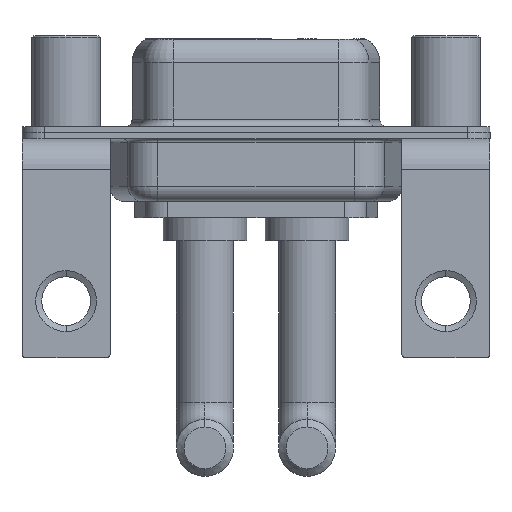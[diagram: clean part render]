
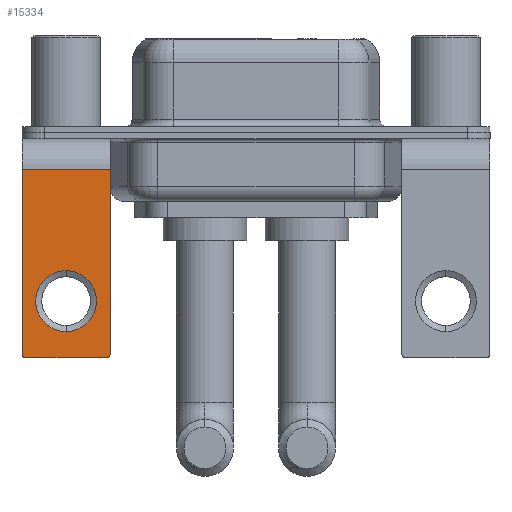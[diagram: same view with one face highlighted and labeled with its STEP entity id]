
A CAD part, front view. The second image highlights one B-rep face of the part: STEP entity #15334.
In plain terms, the highlighted planar face has unit normal (0, -1, 0).
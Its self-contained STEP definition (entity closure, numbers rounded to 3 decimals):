
#143 = CARTESIAN_POINT ( 'NONE',  ( -2.9, -6.25, -14.55 ) ) ;
#316 = CARTESIAN_POINT ( 'NONE',  ( 2.9, -6.25, -2.4 ) ) ;
#358 = ORIENTED_EDGE ( 'NONE', *, *, #3261, .T. ) ;
#514 = DIRECTION ( 'NONE',  ( 0., 0., 1. ) ) ;
#973 = VERTEX_POINT ( 'NONE', #11281 ) ;
#980 = CIRCLE ( 'NONE', #6092, 0.25 ) ;
#1314 = VECTOR ( 'NONE', #4201, 1000. ) ;
#1320 = VECTOR ( 'NONE', #4172, 1000. ) ;
#1619 = DIRECTION ( 'NONE',  ( -1., 0., 0. ) ) ;
#1634 = AXIS2_PLACEMENT_3D ( 'NONE', #6659, #12765, #7776 ) ;
#1833 = CARTESIAN_POINT ( 'NONE',  ( 0., -6.25, -11.07 ) ) ;
#1872 = CARTESIAN_POINT ( 'NONE',  ( -2.9, -6.25, -2.4 ) ) ;
#1983 = CARTESIAN_POINT ( 'NONE',  ( 2.65, -6.25, -14.8 ) ) ;
#2812 = VERTEX_POINT ( 'NONE', #143 ) ;
#3261 = EDGE_CURVE ( 'NONE', #2812, #8365, #980, .T. ) ;
#4140 = VECTOR ( 'NONE', #1619, 1000. ) ;
#4163 = FACE_BOUND ( 'NONE', #8714, .T. ) ;
#4172 = DIRECTION ( 'NONE',  ( 0., 0., -1. ) ) ;
#4201 = DIRECTION ( 'NONE',  ( -1., 0., 0. ) ) ;
#4545 = EDGE_CURVE ( 'NONE', #973, #2812, #15182, .T. ) ;
#4683 = AXIS2_PLACEMENT_3D ( 'NONE', #1833, #15303, #13061 ) ;
#4737 = EDGE_LOOP ( 'NONE', ( #15583, #358, #13802, #5341, #8383, #10522 ) ) ;
#4796 = DIRECTION ( 'NONE',  ( 0., -1., 0. ) ) ;
#5288 = EDGE_CURVE ( 'NONE', #7611, #15326, #15635, .T. ) ;
#5341 = ORIENTED_EDGE ( 'NONE', *, *, #14428, .T. ) ;
#5610 = EDGE_CURVE ( 'NONE', #14534, #8365, #6503, .T. ) ;
#5647 = EDGE_CURVE ( 'NONE', #5901, #12718, #8306, .T. ) ;
#5901 = VERTEX_POINT ( 'NONE', #11033 ) ;
#5910 = CARTESIAN_POINT ( 'NONE',  ( 2.9, -6.25, -14.55 ) ) ;
#5926 = CARTESIAN_POINT ( 'NONE',  ( 0., -6.25, -11.07 ) ) ;
#6048 = DIRECTION ( 'NONE',  ( 0., 0., -1. ) ) ;
#6092 = AXIS2_PLACEMENT_3D ( 'NONE', #9459, #4796, #14524 ) ;
#6503 = LINE ( 'NONE', #13732, #4140 ) ;
#6659 = CARTESIAN_POINT ( 'NONE',  ( 2.65, -6.25, -14.55 ) ) ;
#6834 = DIRECTION ( 'NONE',  ( 0., 1., 0. ) ) ;
#7110 = CARTESIAN_POINT ( 'NONE',  ( 0., -6.25, -9.07 ) ) ;
#7523 = ORIENTED_EDGE ( 'NONE', *, *, #5288, .T. ) ;
#7611 = VERTEX_POINT ( 'NONE', #7110 ) ;
#7776 = DIRECTION ( 'NONE',  ( 0., 0., 1. ) ) ;
#8037 = CIRCLE ( 'NONE', #4683, 2. ) ;
#8306 = LINE ( 'NONE', #9587, #15433 ) ;
#8365 = VERTEX_POINT ( 'NONE', #8973 ) ;
#8383 = ORIENTED_EDGE ( 'NONE', *, *, #5647, .F. ) ;
#8704 = AXIS2_PLACEMENT_3D ( 'NONE', #5926, #6834, #15500 ) ;
#8714 = EDGE_LOOP ( 'NONE', ( #12836, #7523 ) ) ;
#8802 = AXIS2_PLACEMENT_3D ( 'NONE', #9298, #11482, #514 ) ;
#8973 = CARTESIAN_POINT ( 'NONE',  ( -2.65, -6.25, -14.8 ) ) ;
#9298 = CARTESIAN_POINT ( 'NONE',  ( 2.9, -6.25, -2.4 ) ) ;
#9459 = CARTESIAN_POINT ( 'NONE',  ( -2.65, -6.25, -14.55 ) ) ;
#9587 = CARTESIAN_POINT ( 'NONE',  ( 2.9, -6.25, -2.4 ) ) ;
#9976 = EDGE_CURVE ( 'NONE', #5901, #973, #11442, .T. ) ;
#10522 = ORIENTED_EDGE ( 'NONE', *, *, #9976, .T. ) ;
#11033 = CARTESIAN_POINT ( 'NONE',  ( 2.9, -6.25, -2.4 ) ) ;
#11281 = CARTESIAN_POINT ( 'NONE',  ( -2.9, -6.25, -2.4 ) ) ;
#11407 = FACE_OUTER_BOUND ( 'NONE', #4737, .T. ) ;
#11442 = LINE ( 'NONE', #316, #1314 ) ;
#11482 = DIRECTION ( 'NONE',  ( 0., 1., 0. ) ) ;
#11723 = PLANE ( 'NONE',  #8802 ) ;
#12121 = CIRCLE ( 'NONE', #1634, 0.25 ) ;
#12718 = VERTEX_POINT ( 'NONE', #5910 ) ;
#12765 = DIRECTION ( 'NONE',  ( 0., -1., 0. ) ) ;
#12836 = ORIENTED_EDGE ( 'NONE', *, *, #13004, .T. ) ;
#13004 = EDGE_CURVE ( 'NONE', #15326, #7611, #8037, .T. ) ;
#13061 = DIRECTION ( 'NONE',  ( 0., 0., 1. ) ) ;
#13732 = CARTESIAN_POINT ( 'NONE',  ( 2.9, -6.25, -14.8 ) ) ;
#13802 = ORIENTED_EDGE ( 'NONE', *, *, #5610, .F. ) ;
#14428 = EDGE_CURVE ( 'NONE', #14534, #12718, #12121, .T. ) ;
#14524 = DIRECTION ( 'NONE',  ( 0., 0., 1. ) ) ;
#14534 = VERTEX_POINT ( 'NONE', #1983 ) ;
#15182 = LINE ( 'NONE', #1872, #1320 ) ;
#15303 = DIRECTION ( 'NONE',  ( 0., 1., 0. ) ) ;
#15326 = VERTEX_POINT ( 'NONE', #15411 ) ;
#15334 = ADVANCED_FACE ( 'NONE', ( #4163, #11407 ), #11723, .F. ) ;
#15411 = CARTESIAN_POINT ( 'NONE',  ( 0., -6.25, -13.07 ) ) ;
#15433 = VECTOR ( 'NONE', #6048, 1000. ) ;
#15500 = DIRECTION ( 'NONE',  ( 0., 0., 1. ) ) ;
#15583 = ORIENTED_EDGE ( 'NONE', *, *, #4545, .T. ) ;
#15635 = CIRCLE ( 'NONE', #8704, 2. ) ;
